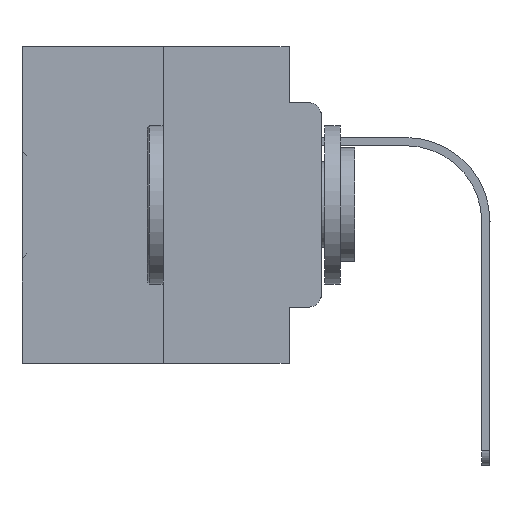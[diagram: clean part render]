
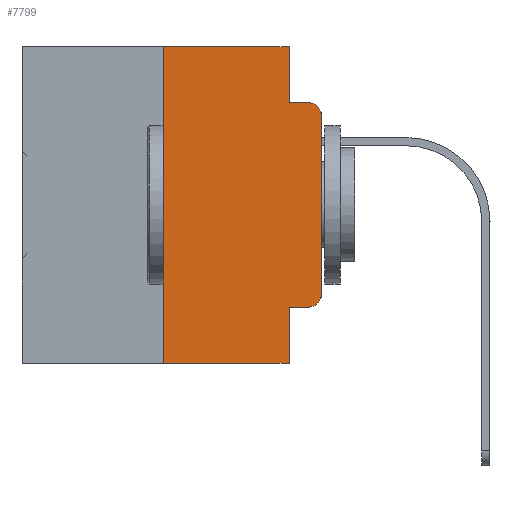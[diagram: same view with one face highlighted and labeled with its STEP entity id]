
A CAD part, left-side view. The second image highlights one B-rep face of the part: STEP entity #7799.
In plain terms, the highlighted planar face has unit normal (-1, 0, 0).
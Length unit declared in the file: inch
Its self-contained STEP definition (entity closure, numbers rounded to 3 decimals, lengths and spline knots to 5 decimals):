
#948 = DIRECTION ( 'NONE',  ( -1., 0., 0. ) ) ;
#1218 = EDGE_CURVE ( 'NONE', #13361, #7163, #28960, .T. ) ;
#1304 = CARTESIAN_POINT ( 'NONE',  ( 0., 0.051, 0. ) ) ;
#1336 = EDGE_CURVE ( 'NONE', #32161, #18287, #6564, .T. ) ;
#2237 = ORIENTED_EDGE ( 'NONE', *, *, #32186, .F. ) ;
#2373 = PLANE ( 'NONE',  #15272 ) ;
#2376 = ORIENTED_EDGE ( 'NONE', *, *, #5329, .F. ) ;
#2613 = VECTOR ( 'NONE', #11655, 39.37008 ) ;
#2820 = CARTESIAN_POINT ( 'NONE',  ( 0., 0.051, -0.0885 ) ) ;
#2875 = CIRCLE ( 'NONE', #26170, 0.02 ) ;
#2982 = VECTOR ( 'NONE', #4212, 39.37008 ) ;
#2983 = LINE ( 'NONE', #20025, #21322 ) ;
#3209 = VERTEX_POINT ( 'NONE', #26505 ) ;
#4185 = DIRECTION ( 'NONE',  ( 0., 0., 1. ) ) ;
#4212 = DIRECTION ( 'NONE',  ( 0., -1., 0. ) ) ;
#4353 = CARTESIAN_POINT ( 'NONE',  ( 0., 0., 0. ) ) ;
#4707 = LINE ( 'NONE', #27952, #2982 ) ;
#4813 = DIRECTION ( 'NONE',  ( 0., 0., 1. ) ) ;
#5329 = EDGE_CURVE ( 'NONE', #31562, #13361, #2983, .T. ) ;
#6013 = ORIENTED_EDGE ( 'NONE', *, *, #1218, .F. ) ;
#6207 = EDGE_LOOP ( 'NONE', ( #12131, #9007, #23180, #6013, #2376, #2237, #8771, #9625, #15753, #21485 ) ) ;
#6564 = LINE ( 'NONE', #4353, #28495 ) ;
#7163 = VERTEX_POINT ( 'NONE', #2820 ) ;
#7799 = ADVANCED_FACE ( 'NONE', ( #26119 ), #2373, .F. ) ;
#7839 = VECTOR ( 'NONE', #4813, 39.37008 ) ;
#7965 = DIRECTION ( 'NONE',  ( 0., 0., -1. ) ) ;
#8771 = ORIENTED_EDGE ( 'NONE', *, *, #13086, .T. ) ;
#9007 = ORIENTED_EDGE ( 'NONE', *, *, #10959, .T. ) ;
#9115 = CARTESIAN_POINT ( 'NONE',  ( 0., 0.02, -0.4115 ) ) ;
#9625 = ORIENTED_EDGE ( 'NONE', *, *, #14752, .F. ) ;
#10784 = DIRECTION ( 'NONE',  ( 0., -1., 0. ) ) ;
#10959 = EDGE_CURVE ( 'NONE', #18287, #25385, #2875, .T. ) ;
#11655 = DIRECTION ( 'NONE',  ( 0., 0., -1. ) ) ;
#12131 = ORIENTED_EDGE ( 'NONE', *, *, #1336, .T. ) ;
#12388 = CARTESIAN_POINT ( 'NONE',  ( 0., 0.02, -0.0885 ) ) ;
#12391 = DIRECTION ( 'NONE',  ( 1., 0., 0. ) ) ;
#12406 = EDGE_CURVE ( 'NONE', #7163, #25385, #31891, .T. ) ;
#13086 = EDGE_CURVE ( 'NONE', #24137, #29596, #17288, .T. ) ;
#13361 = VERTEX_POINT ( 'NONE', #14378 ) ;
#14378 = CARTESIAN_POINT ( 'NONE',  ( 0., 0.051, 0. ) ) ;
#14752 = EDGE_CURVE ( 'NONE', #3209, #29596, #24550, .T. ) ;
#14753 = DIRECTION ( 'NONE',  ( 0., -1., 0. ) ) ;
#15158 = AXIS2_PLACEMENT_3D ( 'NONE', #24358, #948, #32317 ) ;
#15272 = AXIS2_PLACEMENT_3D ( 'NONE', #15278, #12391, #7965 ) ;
#15278 = CARTESIAN_POINT ( 'NONE',  ( 0., 0.473, 0. ) ) ;
#15627 = CARTESIAN_POINT ( 'NONE',  ( 0., 0.051, -0.5 ) ) ;
#15753 = ORIENTED_EDGE ( 'NONE', *, *, #33084, .T. ) ;
#15923 = VERTEX_POINT ( 'NONE', #9115 ) ;
#17288 = LINE ( 'NONE', #27615, #27968 ) ;
#17601 = CARTESIAN_POINT ( 'NONE',  ( 0., 0.25, 0. ) ) ;
#17722 = LINE ( 'NONE', #28056, #7839 ) ;
#18287 = VERTEX_POINT ( 'NONE', #21215 ) ;
#18881 = CARTESIAN_POINT ( 'NONE',  ( 0., 0.02, -0.1085 ) ) ;
#20025 = CARTESIAN_POINT ( 'NONE',  ( 0., 0.473, 0. ) ) ;
#20596 = CARTESIAN_POINT ( 'NONE',  ( 0., 0., -0.3915 ) ) ;
#21103 = VECTOR ( 'NONE', #23563, 39.37008 ) ;
#21215 = CARTESIAN_POINT ( 'NONE',  ( 0., 0., -0.1085 ) ) ;
#21322 = VECTOR ( 'NONE', #10784, 39.37008 ) ;
#21485 = ORIENTED_EDGE ( 'NONE', *, *, #22167, .T. ) ;
#22167 = EDGE_CURVE ( 'NONE', #15923, #32161, #28679, .T. ) ;
#23180 = ORIENTED_EDGE ( 'NONE', *, *, #12406, .F. ) ;
#23563 = DIRECTION ( 'NONE',  ( 0., 0., -1. ) ) ;
#24053 = CARTESIAN_POINT ( 'NONE',  ( 0., 0.051, 0. ) ) ;
#24137 = VERTEX_POINT ( 'NONE', #26161 ) ;
#24358 = CARTESIAN_POINT ( 'NONE',  ( 0., 0.02, -0.3915 ) ) ;
#24550 = LINE ( 'NONE', #1304, #2613 ) ;
#25385 = VERTEX_POINT ( 'NONE', #12388 ) ;
#25712 = VECTOR ( 'NONE', #29703, 39.37008 ) ;
#26119 = FACE_OUTER_BOUND ( 'NONE', #6207, .T. ) ;
#26161 = CARTESIAN_POINT ( 'NONE',  ( 0., 0.25, -0.5 ) ) ;
#26170 = AXIS2_PLACEMENT_3D ( 'NONE', #18881, #29214, #31263 ) ;
#26505 = CARTESIAN_POINT ( 'NONE',  ( 0., 0.051, -0.4115 ) ) ;
#27615 = CARTESIAN_POINT ( 'NONE',  ( 0., 0.473, -0.5 ) ) ;
#27952 = CARTESIAN_POINT ( 'NONE',  ( 0., 0.051, -0.4115 ) ) ;
#27968 = VECTOR ( 'NONE', #14753, 39.37008 ) ;
#28056 = CARTESIAN_POINT ( 'NONE',  ( 0., 0.25, 0. ) ) ;
#28495 = VECTOR ( 'NONE', #4185, 39.37008 ) ;
#28679 = CIRCLE ( 'NONE', #15158, 0.02 ) ;
#28960 = LINE ( 'NONE', #24053, #21103 ) ;
#29214 = DIRECTION ( 'NONE',  ( -1., 0., 0. ) ) ;
#29358 = CARTESIAN_POINT ( 'NONE',  ( 0., 0.051, -0.0885 ) ) ;
#29596 = VERTEX_POINT ( 'NONE', #15627 ) ;
#29703 = DIRECTION ( 'NONE',  ( 0., -1., 0. ) ) ;
#31263 = DIRECTION ( 'NONE',  ( 0., 0., -1. ) ) ;
#31562 = VERTEX_POINT ( 'NONE', #17601 ) ;
#31891 = LINE ( 'NONE', #29358, #25712 ) ;
#32161 = VERTEX_POINT ( 'NONE', #20596 ) ;
#32186 = EDGE_CURVE ( 'NONE', #24137, #31562, #17722, .T. ) ;
#32317 = DIRECTION ( 'NONE',  ( 0., 0., -1. ) ) ;
#33084 = EDGE_CURVE ( 'NONE', #3209, #15923, #4707, .T. ) ;
